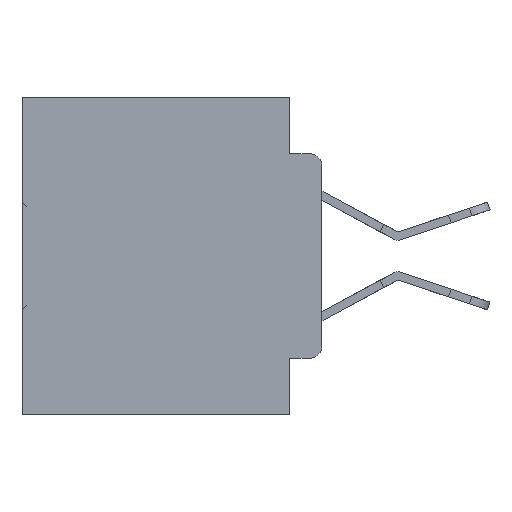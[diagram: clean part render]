
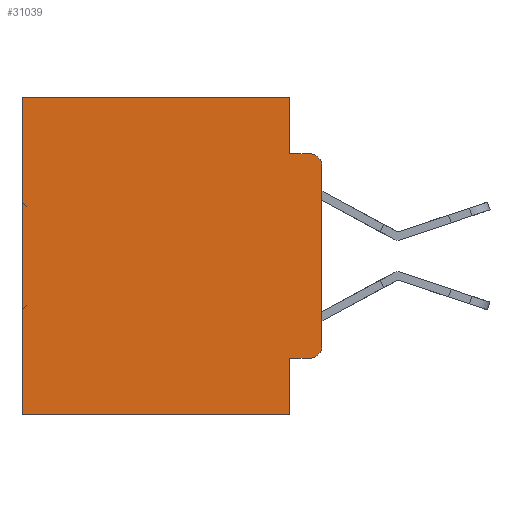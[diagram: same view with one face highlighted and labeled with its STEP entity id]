
A CAD part, left-side view. The second image highlights one B-rep face of the part: STEP entity #31039.
In plain terms, the highlighted planar face has unit normal (-1, 0, 0).
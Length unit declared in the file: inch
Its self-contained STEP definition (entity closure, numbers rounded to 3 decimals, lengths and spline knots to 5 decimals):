
#1353 = VERTEX_POINT ( 'NONE', #14878 ) ;
#1984 = EDGE_CURVE ( 'NONE', #7392, #32750, #13048, .T. ) ;
#2261 = EDGE_CURVE ( 'NONE', #9893, #1353, #22601, .T. ) ;
#2589 = VECTOR ( 'NONE', #29328, 39.37008 ) ;
#3313 = CARTESIAN_POINT ( 'NONE',  ( 0.298, 0.02, -0.3915 ) ) ;
#3360 = VERTEX_POINT ( 'NONE', #5557 ) ;
#3466 = AXIS2_PLACEMENT_3D ( 'NONE', #18334, #18708, #27534 ) ;
#3590 = DIRECTION ( 'NONE',  ( 1., 0., 0. ) ) ;
#3835 = FACE_OUTER_BOUND ( 'NONE', #28549, .T. ) ;
#4170 = CARTESIAN_POINT ( 'NONE',  ( 0.298, 0.02, -0.0885 ) ) ;
#4350 = CARTESIAN_POINT ( 'NONE',  ( 0.298, 0., -0.5 ) ) ;
#4551 = CARTESIAN_POINT ( 'NONE',  ( 0.298, 0.473, -0.5 ) ) ;
#5557 = CARTESIAN_POINT ( 'NONE',  ( 0.298, 0.02, -0.4115 ) ) ;
#5941 = DIRECTION ( 'NONE',  ( 0., 0., -1. ) ) ;
#6353 = DIRECTION ( 'NONE',  ( 0., 0., -1. ) ) ;
#6798 = CARTESIAN_POINT ( 'NONE',  ( 0.298, 0.473, 0. ) ) ;
#7160 = CARTESIAN_POINT ( 'NONE',  ( 0.298, 0.051, -0.0885 ) ) ;
#7392 = VERTEX_POINT ( 'NONE', #35266 ) ;
#7414 = DIRECTION ( 'NONE',  ( 0., -1., 0. ) ) ;
#7768 = CARTESIAN_POINT ( 'NONE',  ( 0.298, 0., -0.3915 ) ) ;
#7816 = ORIENTED_EDGE ( 'NONE', *, *, #36827, .T. ) ;
#8902 = VECTOR ( 'NONE', #19499, 39.37008 ) ;
#9415 = PLANE ( 'NONE',  #25565 ) ;
#9836 = CARTESIAN_POINT ( 'NONE',  ( 0.298, 0., 0. ) ) ;
#9893 = VERTEX_POINT ( 'NONE', #21294 ) ;
#11015 = VERTEX_POINT ( 'NONE', #12092 ) ;
#11307 = ORIENTED_EDGE ( 'NONE', *, *, #37415, .F. ) ;
#11469 = LINE ( 'NONE', #6798, #24725 ) ;
#11856 = VERTEX_POINT ( 'NONE', #4170 ) ;
#12092 = CARTESIAN_POINT ( 'NONE',  ( 0.298, 0.051, -0.4115 ) ) ;
#13014 = LINE ( 'NONE', #7160, #28081 ) ;
#13048 = LINE ( 'NONE', #35671, #2589 ) ;
#13968 = EDGE_CURVE ( 'NONE', #7392, #11856, #27490, .T. ) ;
#14878 = CARTESIAN_POINT ( 'NONE',  ( 0.298, 0.051, -0.0885 ) ) ;
#15036 = ORIENTED_EDGE ( 'NONE', *, *, #21945, .T. ) ;
#16387 = ORIENTED_EDGE ( 'NONE', *, *, #21920, .T. ) ;
#18334 = CARTESIAN_POINT ( 'NONE',  ( 0.298, 0.02, -0.1085 ) ) ;
#18476 = CARTESIAN_POINT ( 'NONE',  ( 0.298, 0.051, -0.4115 ) ) ;
#18708 = DIRECTION ( 'NONE',  ( -1., 0., 0. ) ) ;
#19066 = ORIENTED_EDGE ( 'NONE', *, *, #2261, .F. ) ;
#19226 = VERTEX_POINT ( 'NONE', #19660 ) ;
#19499 = DIRECTION ( 'NONE',  ( 0., 0., -1. ) ) ;
#19510 = ORIENTED_EDGE ( 'NONE', *, *, #27430, .T. ) ;
#19660 = CARTESIAN_POINT ( 'NONE',  ( 0.298, 0.473, 0. ) ) ;
#19822 = VERTEX_POINT ( 'NONE', #23383 ) ;
#20115 = LINE ( 'NONE', #18476, #24244 ) ;
#20624 = ORIENTED_EDGE ( 'NONE', *, *, #27501, .F. ) ;
#21106 = DIRECTION ( 'NONE',  ( -1., 0., 0. ) ) ;
#21134 = DIRECTION ( 'NONE',  ( 0., 0., -1. ) ) ;
#21294 = CARTESIAN_POINT ( 'NONE',  ( 0.298, 0.051, 0. ) ) ;
#21326 = ORIENTED_EDGE ( 'NONE', *, *, #1984, .F. ) ;
#21524 = VERTEX_POINT ( 'NONE', #4551 ) ;
#21564 = DIRECTION ( 'NONE',  ( 0., 1., 0. ) ) ;
#21920 = EDGE_CURVE ( 'NONE', #19226, #21524, #11469, .T. ) ;
#21945 = EDGE_CURVE ( 'NONE', #11015, #3360, #20115, .T. ) ;
#22155 = LINE ( 'NONE', #23380, #28958 ) ;
#22601 = LINE ( 'NONE', #31457, #8902 ) ;
#23380 = CARTESIAN_POINT ( 'NONE',  ( 0.298, 0.051, 0. ) ) ;
#23383 = CARTESIAN_POINT ( 'NONE',  ( 0.298, 0.051, -0.5 ) ) ;
#23994 = DIRECTION ( 'NONE',  ( 0., 0., -1. ) ) ;
#24244 = VECTOR ( 'NONE', #24374, 39.37008 ) ;
#24339 = DIRECTION ( 'NONE',  ( 0., 1., 0. ) ) ;
#24374 = DIRECTION ( 'NONE',  ( 0., -1., 0. ) ) ;
#24725 = VECTOR ( 'NONE', #23994, 39.37008 ) ;
#24900 = VECTOR ( 'NONE', #21564, 39.37008 ) ;
#25238 = EDGE_CURVE ( 'NONE', #19822, #21524, #26919, .T. ) ;
#25565 = AXIS2_PLACEMENT_3D ( 'NONE', #29753, #3590, #21134 ) ;
#25819 = LINE ( 'NONE', #9836, #24900 ) ;
#26919 = LINE ( 'NONE', #4350, #30960 ) ;
#27430 = EDGE_CURVE ( 'NONE', #9893, #19226, #25819, .T. ) ;
#27490 = CIRCLE ( 'NONE', #3466, 0.02 ) ;
#27501 = EDGE_CURVE ( 'NONE', #1353, #11856, #13014, .T. ) ;
#27534 = DIRECTION ( 'NONE',  ( 0., 0., -1. ) ) ;
#27625 = AXIS2_PLACEMENT_3D ( 'NONE', #3313, #21106, #6353 ) ;
#28081 = VECTOR ( 'NONE', #7414, 39.37008 ) ;
#28549 = EDGE_LOOP ( 'NONE', ( #21326, #31163, #20624, #19066, #19510, #16387, #37038, #11307, #15036, #7816 ) ) ;
#28958 = VECTOR ( 'NONE', #5941, 39.37008 ) ;
#29328 = DIRECTION ( 'NONE',  ( 0., 0., -1. ) ) ;
#29753 = CARTESIAN_POINT ( 'NONE',  ( 0.298, 0., 0. ) ) ;
#30960 = VECTOR ( 'NONE', #24339, 39.37008 ) ;
#31039 = ADVANCED_FACE ( 'NONE', ( #3835 ), #9415, .F. ) ;
#31163 = ORIENTED_EDGE ( 'NONE', *, *, #13968, .T. ) ;
#31457 = CARTESIAN_POINT ( 'NONE',  ( 0.298, 0.051, 0. ) ) ;
#32750 = VERTEX_POINT ( 'NONE', #7768 ) ;
#33984 = CIRCLE ( 'NONE', #27625, 0.02 ) ;
#35266 = CARTESIAN_POINT ( 'NONE',  ( 0.298, 0., -0.1085 ) ) ;
#35671 = CARTESIAN_POINT ( 'NONE',  ( 0.298, 0., 0. ) ) ;
#36827 = EDGE_CURVE ( 'NONE', #3360, #32750, #33984, .T. ) ;
#37038 = ORIENTED_EDGE ( 'NONE', *, *, #25238, .F. ) ;
#37415 = EDGE_CURVE ( 'NONE', #11015, #19822, #22155, .T. ) ;
